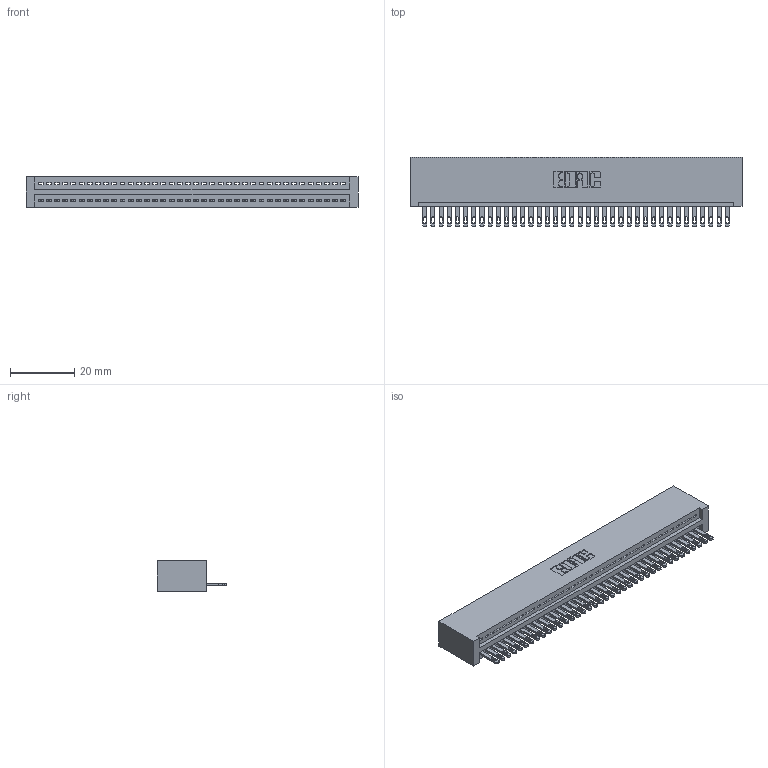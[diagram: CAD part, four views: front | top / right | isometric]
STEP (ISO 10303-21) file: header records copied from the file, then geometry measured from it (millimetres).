
FILE_DESCRIPTION (( 'STEP AP203' ), '1' );
FILE_NAME ('895-038-500-101.STEP', '2020-09-26T00:44:02', ( '' ), ( '' ), 'SwSTEP 2.0', 'SolidWorks 2020', '' );
FILE_SCHEMA (( 'CONFIG_CONTROL_DESIGN' ));
Length unit declared in the file: inch
Products named in the file (3): 345-292-001_345-293-100; 895-038-500-101; 845 Part_No Mounting Lugs
Assembly tree (39 placements, depth 2):
  895-038-500-101
    845 Part_No Mounting Lugs
    345-292-001_345-293-100  x38
Bounding box: 103.12 x 21.51 x 9.4 mm (x, y, z)
Volume: 10369.9 mm3; surface area: 14001.8 mm2
Topology: 39 solids, 39 shells, 2170 faces, 6701 edges, 4466 vertices
Faces by surface type: plane 1368, cylinder 802
Entity records: 28791 total; most frequent: CARTESIAN_POINT 4994, ORIENTED_EDGE 4966, DIRECTION 4363, EDGE_CURVE 2483, VECTOR 2203, LINE 2203, VERTEX_POINT 1654, AXIS2_PLACEMENT_3D 1080
